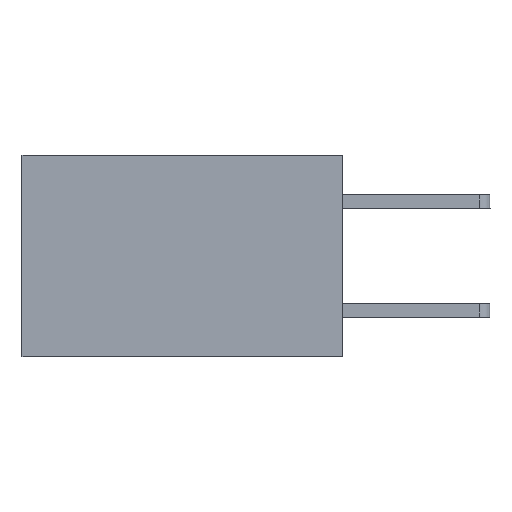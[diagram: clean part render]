
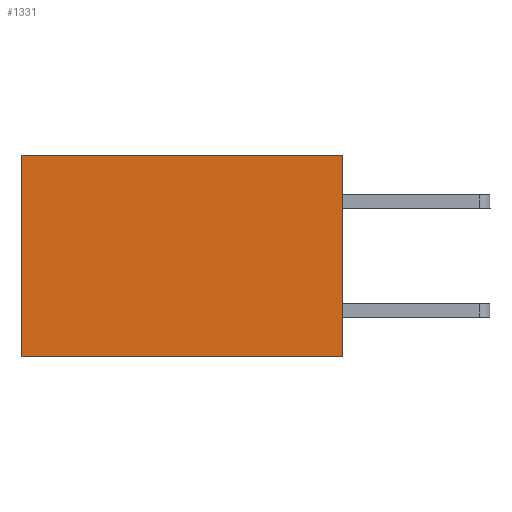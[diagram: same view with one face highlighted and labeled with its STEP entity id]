
A CAD part, left-side view. The second image highlights one B-rep face of the part: STEP entity #1331.
In plain terms, the highlighted planar face has unit normal (-1, 0, 0).
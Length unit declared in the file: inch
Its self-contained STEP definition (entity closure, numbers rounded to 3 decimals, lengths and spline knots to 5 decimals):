
#202 = EDGE_CURVE ( 'NONE', #5539, #1354, #5197, .T. ) ;
#375 = CARTESIAN_POINT ( 'NONE',  ( 0.277, 0., -0.37 ) ) ;
#516 = CARTESIAN_POINT ( 'NONE',  ( 0.277, 0.59, 0. ) ) ;
#554 = ORIENTED_EDGE ( 'NONE', *, *, #202, .F. ) ;
#898 = DIRECTION ( 'NONE',  ( 0., 0., -1. ) ) ;
#1013 = CARTESIAN_POINT ( 'NONE',  ( 0.277, 0.59, -0.37 ) ) ;
#1331 = ADVANCED_FACE ( 'NONE', ( #7163 ), #7751, .F. ) ;
#1354 = VERTEX_POINT ( 'NONE', #7478 ) ;
#1469 = CARTESIAN_POINT ( 'NONE',  ( 0.277, 0., -0.37 ) ) ;
#2469 = VECTOR ( 'NONE', #898, 39.37008 ) ;
#2517 = ORIENTED_EDGE ( 'NONE', *, *, #4545, .T. ) ;
#3548 = VECTOR ( 'NONE', #7834, 39.37008 ) ;
#3735 = EDGE_LOOP ( 'NONE', ( #5787, #7436, #554, #2517 ) ) ;
#4196 = CARTESIAN_POINT ( 'NONE',  ( 0.277, 0.59, -0.37 ) ) ;
#4262 = LINE ( 'NONE', #1013, #2469 ) ;
#4281 = DIRECTION ( 'NONE',  ( 0., 1., 0. ) ) ;
#4369 = CARTESIAN_POINT ( 'NONE',  ( 0.277, 0., 0. ) ) ;
#4545 = EDGE_CURVE ( 'NONE', #5539, #5261, #6733, .T. ) ;
#4756 = VECTOR ( 'NONE', #6749, 39.37008 ) ;
#5020 = VECTOR ( 'NONE', #4281, 39.37008 ) ;
#5140 = EDGE_CURVE ( 'NONE', #5261, #7086, #4262, .T. ) ;
#5197 = LINE ( 'NONE', #375, #3548 ) ;
#5261 = VERTEX_POINT ( 'NONE', #516 ) ;
#5539 = VERTEX_POINT ( 'NONE', #7334 ) ;
#5787 = ORIENTED_EDGE ( 'NONE', *, *, #5140, .T. ) ;
#6733 = LINE ( 'NONE', #4369, #5020 ) ;
#6749 = DIRECTION ( 'NONE',  ( 0., 1., 0. ) ) ;
#7086 = VERTEX_POINT ( 'NONE', #4196 ) ;
#7163 = FACE_OUTER_BOUND ( 'NONE', #3735, .T. ) ;
#7254 = DIRECTION ( 'NONE',  ( 0., 0., -1. ) ) ;
#7334 = CARTESIAN_POINT ( 'NONE',  ( 0.277, 0., 0. ) ) ;
#7372 = DIRECTION ( 'NONE',  ( 1., 0., 0. ) ) ;
#7436 = ORIENTED_EDGE ( 'NONE', *, *, #8102, .F. ) ;
#7478 = CARTESIAN_POINT ( 'NONE',  ( 0.277, 0., -0.37 ) ) ;
#7714 = CARTESIAN_POINT ( 'NONE',  ( 0.277, 0., -0.37 ) ) ;
#7751 = PLANE ( 'NONE',  #7759 ) ;
#7759 = AXIS2_PLACEMENT_3D ( 'NONE', #7714, #7372, #7254 ) ;
#7834 = DIRECTION ( 'NONE',  ( 0., 0., -1. ) ) ;
#8102 = EDGE_CURVE ( 'NONE', #1354, #7086, #8510, .T. ) ;
#8510 = LINE ( 'NONE', #1469, #4756 ) ;
